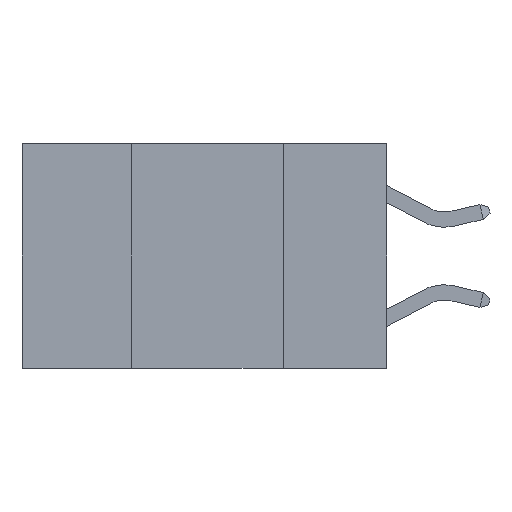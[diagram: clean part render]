
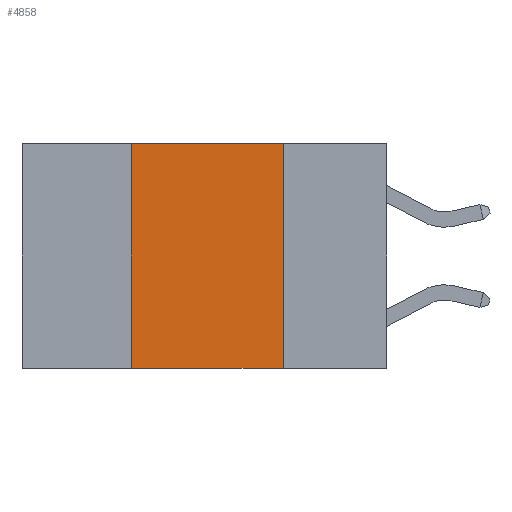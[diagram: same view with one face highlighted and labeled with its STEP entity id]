
A CAD part, left-side view. The second image highlights one B-rep face of the part: STEP entity #4858.
In plain terms, the highlighted planar face has unit normal (-1, 0, 0).
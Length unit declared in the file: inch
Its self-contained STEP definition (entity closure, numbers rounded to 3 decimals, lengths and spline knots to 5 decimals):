
#281 = DIRECTION ( 'NONE',  ( 0., 0., -1. ) ) ;
#594 = CARTESIAN_POINT ( 'NONE',  ( 0., 0.6, -0.37 ) ) ;
#2013 = VERTEX_POINT ( 'NONE', #7077 ) ;
#2062 = VECTOR ( 'NONE', #5891, 39.37008 ) ;
#2100 = ORIENTED_EDGE ( 'NONE', *, *, #6196, .F. ) ;
#2372 = VERTEX_POINT ( 'NONE', #3477 ) ;
#2612 = CARTESIAN_POINT ( 'NONE',  ( 0., 0.42, 0. ) ) ;
#2616 = AXIS2_PLACEMENT_3D ( 'NONE', #7623, #6627, #281 ) ;
#2649 = CARTESIAN_POINT ( 'NONE',  ( 0., 0.42, -0.37 ) ) ;
#3477 = CARTESIAN_POINT ( 'NONE',  ( 0., 0.17, -0.37 ) ) ;
#4490 = VERTEX_POINT ( 'NONE', #5971 ) ;
#4493 = LINE ( 'NONE', #9633, #11982 ) ;
#4858 = ADVANCED_FACE ( 'NONE', ( #10033 ), #5530, .F. ) ;
#4927 = ORIENTED_EDGE ( 'NONE', *, *, #10376, .F. ) ;
#5515 = DIRECTION ( 'NONE',  ( 0., -1., 0. ) ) ;
#5519 = VECTOR ( 'NONE', #7867, 39.37008 ) ;
#5530 = PLANE ( 'NONE',  #2616 ) ;
#5891 = DIRECTION ( 'NONE',  ( 0., -1., 0. ) ) ;
#5971 = CARTESIAN_POINT ( 'NONE',  ( 0., 0.42, 0. ) ) ;
#6196 = EDGE_CURVE ( 'NONE', #4490, #2013, #4493, .T. ) ;
#6627 = DIRECTION ( 'NONE',  ( 1., 0., 0. ) ) ;
#7077 = CARTESIAN_POINT ( 'NONE',  ( 0., 0.17, 0. ) ) ;
#7115 = EDGE_LOOP ( 'NONE', ( #10043, #2100, #4927, #7716 ) ) ;
#7623 = CARTESIAN_POINT ( 'NONE',  ( 0., 0.6, 0. ) ) ;
#7679 = LINE ( 'NONE', #8972, #12637 ) ;
#7716 = ORIENTED_EDGE ( 'NONE', *, *, #10441, .T. ) ;
#7867 = DIRECTION ( 'NONE',  ( 0., 0., 1. ) ) ;
#8607 = VERTEX_POINT ( 'NONE', #2649 ) ;
#8972 = CARTESIAN_POINT ( 'NONE',  ( 0., 0.17, 0. ) ) ;
#9633 = CARTESIAN_POINT ( 'NONE',  ( 0., 0.6, 0. ) ) ;
#10033 = FACE_OUTER_BOUND ( 'NONE', #7115, .T. ) ;
#10043 = ORIENTED_EDGE ( 'NONE', *, *, #10438, .F. ) ;
#10376 = EDGE_CURVE ( 'NONE', #8607, #4490, #10971, .T. ) ;
#10438 = EDGE_CURVE ( 'NONE', #2013, #2372, #7679, .T. ) ;
#10441 = EDGE_CURVE ( 'NONE', #8607, #2372, #12939, .T. ) ;
#10971 = LINE ( 'NONE', #2612, #5519 ) ;
#10982 = DIRECTION ( 'NONE',  ( 0., 0., -1. ) ) ;
#11982 = VECTOR ( 'NONE', #5515, 39.37008 ) ;
#12637 = VECTOR ( 'NONE', #10982, 39.37008 ) ;
#12939 = LINE ( 'NONE', #594, #2062 ) ;
